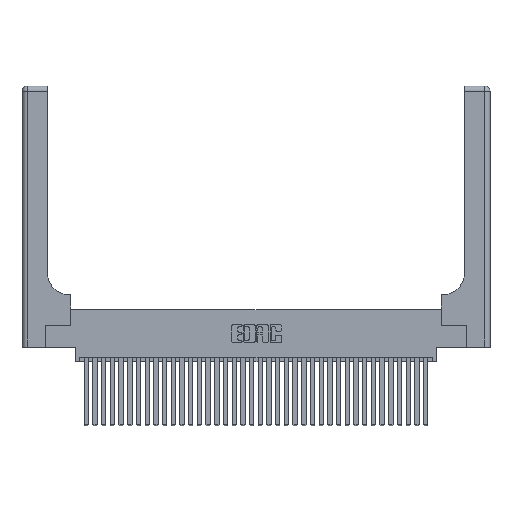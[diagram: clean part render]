
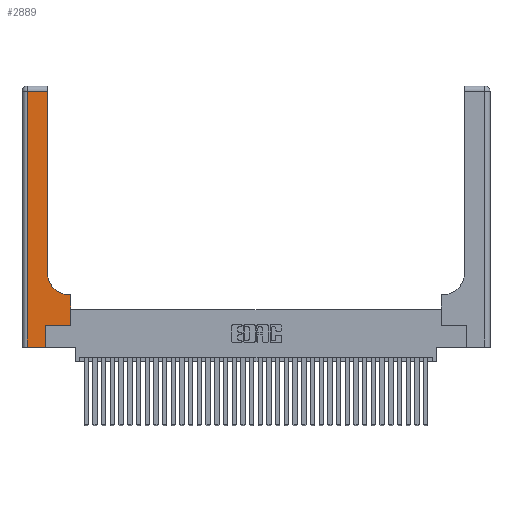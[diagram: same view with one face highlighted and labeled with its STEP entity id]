
A CAD part, top view. The second image highlights one B-rep face of the part: STEP entity #2889.
In plain terms, the highlighted planar face has unit normal (0, 0, 1).
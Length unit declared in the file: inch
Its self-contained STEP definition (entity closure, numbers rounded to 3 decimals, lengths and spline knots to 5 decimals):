
#865 = ORIENTED_EDGE ( 'NONE', *, *, #31329, .T. ) ;
#1714 = LINE ( 'NONE', #1879, #33319 ) ;
#1754 = FACE_OUTER_BOUND ( 'NONE', #14429, .T. ) ;
#1879 = CARTESIAN_POINT ( 'NONE',  ( 0.269, 0., 0.37 ) ) ;
#2530 = CARTESIAN_POINT ( 'NONE',  ( 0.269, 0.25, 0.37 ) ) ;
#2889 = ADVANCED_FACE ( 'NONE', ( #1754 ), #36747, .F. ) ;
#3625 = DIRECTION ( 'NONE',  ( 1., 0., 0. ) ) ;
#6336 = CARTESIAN_POINT ( 'NONE',  ( 0.269, 0.25, 0.37 ) ) ;
#8025 = DIRECTION ( 'NONE',  ( 0., 1., 0. ) ) ;
#8076 = LINE ( 'NONE', #6336, #9779 ) ;
#9779 = VECTOR ( 'NONE', #3625, 39.37008 ) ;
#10893 = VECTOR ( 'NONE', #34728, 39.37008 ) ;
#12021 = CARTESIAN_POINT ( 'NONE',  ( 0.5415, 0.6, 0.37 ) ) ;
#12031 = EDGE_CURVE ( 'NONE', #33260, #35472, #8076, .T. ) ;
#13108 = LINE ( 'NONE', #27012, #26368 ) ;
#13243 = DIRECTION ( 'NONE',  ( -1., 0., 0. ) ) ;
#14429 = EDGE_LOOP ( 'NONE', ( #34848, #15758, #27963, #20548, #20208, #31695, #25927, #865, #27265 ) ) ;
#14614 = EDGE_CURVE ( 'NONE', #19112, #26353, #21566, .T. ) ;
#14676 = CARTESIAN_POINT ( 'NONE',  ( 0.2915, 0.85, 0.37 ) ) ;
#14763 = LINE ( 'NONE', #25237, #32029 ) ;
#14825 = LINE ( 'NONE', #35741, #22417 ) ;
#14860 = CARTESIAN_POINT ( 'NONE',  ( 0.5585, 0.6, 0.37 ) ) ;
#15758 = ORIENTED_EDGE ( 'NONE', *, *, #16509, .T. ) ;
#16218 = VERTEX_POINT ( 'NONE', #20859 ) ;
#16509 = EDGE_CURVE ( 'NONE', #16218, #25588, #13108, .T. ) ;
#16854 = CARTESIAN_POINT ( 'NONE',  ( 0.06, 0., 0.37 ) ) ;
#17052 = LINE ( 'NONE', #34118, #29429 ) ;
#17654 = CARTESIAN_POINT ( 'NONE',  ( 0.269, 0., 0.37 ) ) ;
#19106 = VERTEX_POINT ( 'NONE', #14860 ) ;
#19112 = VERTEX_POINT ( 'NONE', #12021 ) ;
#19166 = CARTESIAN_POINT ( 'NONE',  ( 0.06, 2.94, 0.37 ) ) ;
#19369 = CARTESIAN_POINT ( 'NONE',  ( 0.5415, 0.85, 0.37 ) ) ;
#19924 = DIRECTION ( 'NONE',  ( -1., 0., 0. ) ) ;
#20208 = ORIENTED_EDGE ( 'NONE', *, *, #35191, .T. ) ;
#20548 = ORIENTED_EDGE ( 'NONE', *, *, #32905, .T. ) ;
#20859 = CARTESIAN_POINT ( 'NONE',  ( 0.2915, 2.94, 0.37 ) ) ;
#21566 = CIRCLE ( 'NONE', #36369, 0.25 ) ;
#22377 = DIRECTION ( 'NONE',  ( 0., -1., 0. ) ) ;
#22417 = VECTOR ( 'NONE', #13243, 39.37008 ) ;
#22560 = CARTESIAN_POINT ( 'NONE',  ( 0., 3., 0.37 ) ) ;
#23707 = VERTEX_POINT ( 'NONE', #16854 ) ;
#24175 = AXIS2_PLACEMENT_3D ( 'NONE', #22560, #31103, #19924 ) ;
#25237 = CARTESIAN_POINT ( 'NONE',  ( 0.06, 3., 0.37 ) ) ;
#25588 = VERTEX_POINT ( 'NONE', #19166 ) ;
#25626 = DIRECTION ( 'NONE',  ( 0., 1., 0. ) ) ;
#25927 = ORIENTED_EDGE ( 'NONE', *, *, #31102, .T. ) ;
#25960 = DIRECTION ( 'NONE',  ( 1., 0., 0. ) ) ;
#26353 = VERTEX_POINT ( 'NONE', #14676 ) ;
#26368 = VECTOR ( 'NONE', #32740, 39.37008 ) ;
#27012 = CARTESIAN_POINT ( 'NONE',  ( 0., 2.94, 0.37 ) ) ;
#27039 = VERTEX_POINT ( 'NONE', #17654 ) ;
#27215 = LINE ( 'NONE', #28836, #32064 ) ;
#27265 = ORIENTED_EDGE ( 'NONE', *, *, #14614, .T. ) ;
#27963 = ORIENTED_EDGE ( 'NONE', *, *, #33325, .T. ) ;
#28795 = CARTESIAN_POINT ( 'NONE',  ( 0.5585, 0.25, 0.37 ) ) ;
#28836 = CARTESIAN_POINT ( 'NONE',  ( 0., 0., 0.37 ) ) ;
#29429 = VECTOR ( 'NONE', #25626, 39.37008 ) ;
#30404 = DIRECTION ( 'NONE',  ( 0., 0., -1. ) ) ;
#31102 = EDGE_CURVE ( 'NONE', #35472, #19106, #34849, .T. ) ;
#31103 = DIRECTION ( 'NONE',  ( 0., 0., -1. ) ) ;
#31329 = EDGE_CURVE ( 'NONE', #19106, #19112, #14825, .T. ) ;
#31695 = ORIENTED_EDGE ( 'NONE', *, *, #12031, .T. ) ;
#32029 = VECTOR ( 'NONE', #22377, 39.37008 ) ;
#32064 = VECTOR ( 'NONE', #25960, 39.37008 ) ;
#32740 = DIRECTION ( 'NONE',  ( -1., 0., 0. ) ) ;
#32787 = EDGE_CURVE ( 'NONE', #26353, #16218, #17052, .T. ) ;
#32905 = EDGE_CURVE ( 'NONE', #23707, #27039, #27215, .T. ) ;
#33260 = VERTEX_POINT ( 'NONE', #2530 ) ;
#33319 = VECTOR ( 'NONE', #8025, 39.37008 ) ;
#33325 = EDGE_CURVE ( 'NONE', #25588, #23707, #14763, .T. ) ;
#33565 = DIRECTION ( 'NONE',  ( 1., 0., 0. ) ) ;
#34118 = CARTESIAN_POINT ( 'NONE',  ( 0.2915, 3., 0.37 ) ) ;
#34728 = DIRECTION ( 'NONE',  ( 0., 1., 0. ) ) ;
#34848 = ORIENTED_EDGE ( 'NONE', *, *, #32787, .T. ) ;
#34849 = LINE ( 'NONE', #34956, #10893 ) ;
#34956 = CARTESIAN_POINT ( 'NONE',  ( 0.5585, 0.25, 0.37 ) ) ;
#35191 = EDGE_CURVE ( 'NONE', #27039, #33260, #1714, .T. ) ;
#35472 = VERTEX_POINT ( 'NONE', #28795 ) ;
#35741 = CARTESIAN_POINT ( 'NONE',  ( 0.2915, 0.6, 0.37 ) ) ;
#36369 = AXIS2_PLACEMENT_3D ( 'NONE', #19369, #30404, #33565 ) ;
#36747 = PLANE ( 'NONE',  #24175 ) ;
